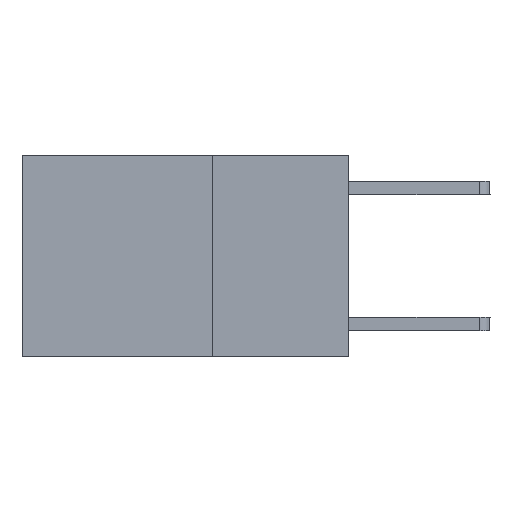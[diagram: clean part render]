
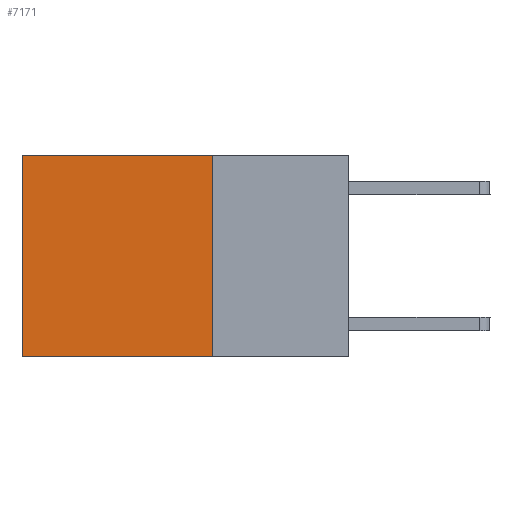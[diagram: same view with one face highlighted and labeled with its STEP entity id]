
A CAD part, left-side view. The second image highlights one B-rep face of the part: STEP entity #7171.
In plain terms, the highlighted planar face has unit normal (-1, 0, 0).
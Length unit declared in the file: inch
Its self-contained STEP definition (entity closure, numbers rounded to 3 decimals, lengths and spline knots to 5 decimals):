
#174 = VECTOR ( 'NONE', #7951, 39.37008 ) ;
#210 = VECTOR ( 'NONE', #8540, 39.37008 ) ;
#553 = CARTESIAN_POINT ( 'NONE',  ( 0.2625, 0.25, 0. ) ) ;
#599 = LINE ( 'NONE', #1484, #3205 ) ;
#703 = ORIENTED_EDGE ( 'NONE', *, *, #6390, .F. ) ;
#878 = CARTESIAN_POINT ( 'NONE',  ( 0.2625, 0.6, -0.37 ) ) ;
#1338 = PLANE ( 'NONE',  #3553 ) ;
#1484 = CARTESIAN_POINT ( 'NONE',  ( 0.2625, 0.25, -0.37 ) ) ;
#1514 = VERTEX_POINT ( 'NONE', #9510 ) ;
#1618 = LINE ( 'NONE', #4121, #174 ) ;
#1871 = CARTESIAN_POINT ( 'NONE',  ( 0.2625, 0.6, 0. ) ) ;
#2058 = DIRECTION ( 'NONE',  ( 0., 1., 0. ) ) ;
#2301 = ORIENTED_EDGE ( 'NONE', *, *, #4835, .T. ) ;
#2799 = VERTEX_POINT ( 'NONE', #878 ) ;
#3162 = EDGE_CURVE ( 'NONE', #3283, #7387, #1618, .T. ) ;
#3163 = DIRECTION ( 'NONE',  ( 0., 0., -1. ) ) ;
#3205 = VECTOR ( 'NONE', #2058, 39.37008 ) ;
#3283 = VERTEX_POINT ( 'NONE', #5820 ) ;
#3553 = AXIS2_PLACEMENT_3D ( 'NONE', #553, #6122, #4536 ) ;
#3747 = LINE ( 'NONE', #10050, #210 ) ;
#3801 = EDGE_LOOP ( 'NONE', ( #2301, #703, #4160, #4019 ) ) ;
#4019 = ORIENTED_EDGE ( 'NONE', *, *, #3162, .T. ) ;
#4121 = CARTESIAN_POINT ( 'NONE',  ( 0.2625, 0.25, 0. ) ) ;
#4160 = ORIENTED_EDGE ( 'NONE', *, *, #7960, .F. ) ;
#4536 = DIRECTION ( 'NONE',  ( 0., 0., -1. ) ) ;
#4835 = EDGE_CURVE ( 'NONE', #7387, #2799, #3747, .T. ) ;
#4899 = CARTESIAN_POINT ( 'NONE',  ( 0.2625, 0.25, 0. ) ) ;
#5337 = FACE_OUTER_BOUND ( 'NONE', #3801, .T. ) ;
#5820 = CARTESIAN_POINT ( 'NONE',  ( 0.2625, 0.25, 0. ) ) ;
#6122 = DIRECTION ( 'NONE',  ( 1., 0., 0. ) ) ;
#6390 = EDGE_CURVE ( 'NONE', #1514, #2799, #599, .T. ) ;
#7171 = ADVANCED_FACE ( 'NONE', ( #5337 ), #1338, .F. ) ;
#7387 = VERTEX_POINT ( 'NONE', #1871 ) ;
#7558 = VECTOR ( 'NONE', #3163, 39.37008 ) ;
#7951 = DIRECTION ( 'NONE',  ( 0., 1., 0. ) ) ;
#7960 = EDGE_CURVE ( 'NONE', #3283, #1514, #9808, .T. ) ;
#8540 = DIRECTION ( 'NONE',  ( 0., 0., -1. ) ) ;
#9510 = CARTESIAN_POINT ( 'NONE',  ( 0.2625, 0.25, -0.37 ) ) ;
#9808 = LINE ( 'NONE', #4899, #7558 ) ;
#10050 = CARTESIAN_POINT ( 'NONE',  ( 0.2625, 0.6, 0. ) ) ;
